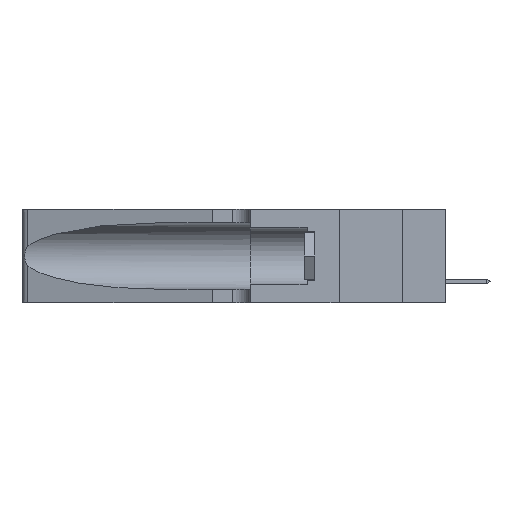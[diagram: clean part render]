
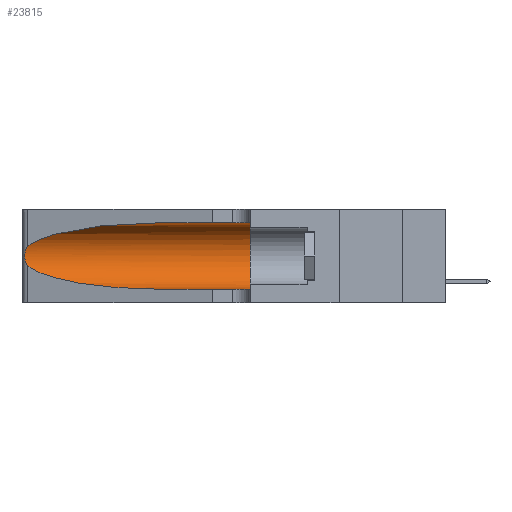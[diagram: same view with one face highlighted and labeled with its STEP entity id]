
A CAD part, left-side view. The second image highlights one B-rep face of the part: STEP entity #23815.
In plain terms, the highlighted cylindrical face has radius 3.308 mm (diameter 6.617 mm), a partial arc.
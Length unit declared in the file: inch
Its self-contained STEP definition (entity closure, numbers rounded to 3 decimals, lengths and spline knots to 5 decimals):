
#308 = CARTESIAN_POINT ( 'NONE',  ( 0.25555, 1.22994, 0.2215 ) ) ;
#346 = EDGE_LOOP ( 'NONE', ( #594, #11282, #1306, #16714, #24257, #5526 ) ) ;
#594 = ORIENTED_EDGE ( 'NONE', *, *, #5024, .T. ) ;
#627 = CARTESIAN_POINT ( 'NONE',  ( 0.26018, 1.23835, 0.19895 ) ) ;
#1306 = ORIENTED_EDGE ( 'NONE', *, *, #1651, .T. ) ;
#1333 = CARTESIAN_POINT ( 'NONE',  ( 0.2373, 1.15595, 0.28018 ) ) ;
#1420 = CARTESIAN_POINT ( 'NONE',  ( 0.25639, 1.23186, 0.15144 ) ) ;
#1492 = CARTESIAN_POINT ( 'NONE',  ( 0.18966, 0.96281, 0.31525 ) ) ;
#1651 = EDGE_CURVE ( 'NONE', #13844, #24138, #10274, .T. ) ;
#1685 = LINE ( 'NONE', #20916, #15355 ) ;
#1821 = CARTESIAN_POINT ( 'NONE',  ( 0.1305, 1.61858, 0.05475 ) ) ;
#2177 = CARTESIAN_POINT ( 'NONE',  ( 0.25789, 1.23486, 0.15765 ) ) ;
#2389 = CARTESIAN_POINT ( 'NONE',  ( 0.1305, 0.35, 0.31525 ) ) ;
#2402 = DIRECTION ( 'NONE',  ( 0., 0., -1. ) ) ;
#3996 = CARTESIAN_POINT ( 'NONE',  ( 0.18966, 0.96281, 0.05475 ) ) ;
#4148 = CARTESIAN_POINT ( 'NONE',  ( 0.25487, 1.22718, 0.14631 ) ) ;
#4607 = VERTEX_POINT ( 'NONE', #18445 ) ;
#4663 = CARTESIAN_POINT ( 'NONE',  ( 0.1305, 0.35, 0.185 ) ) ;
#4810 = EDGE_CURVE ( 'NONE', #20390, #4607, #6855, .T. ) ;
#4836 = DIRECTION ( 'NONE',  ( 0., 0., 1. ) ) ;
#4902 = CARTESIAN_POINT ( 'NONE',  ( 0.25555, 1.22993, 0.14849 ) ) ;
#5024 = EDGE_CURVE ( 'NONE', #6715, #22818, #18009, .T. ) ;
#5433 = DIRECTION ( 'NONE',  ( 0., -1., 0. ) ) ;
#5441 = AXIS2_PLACEMENT_3D ( 'NONE', #4663, #21728, #4836 ) ;
#5526 = ORIENTED_EDGE ( 'NONE', *, *, #13953, .F. ) ;
#5614 = CARTESIAN_POINT ( 'NONE',  ( 0.1305, 0.72297, 0.31525 ) ) ;
#5783 = CARTESIAN_POINT ( 'NONE',  ( 0.25487, 1.22718, 0.22369 ) ) ;
#5871 = CARTESIAN_POINT ( 'NONE',  ( 0.1305, 0.72297, 0.05475 ) ) ;
#6715 = VERTEX_POINT ( 'NONE', #5614 ) ;
#6785 = CARTESIAN_POINT ( 'NONE',  ( 0.1305, 0.72297, 0.05475 ) ) ;
#6855 = CIRCLE ( 'NONE', #5441, 0.13025 ) ;
#8062 = CARTESIAN_POINT ( 'NONE',  ( 0.26075, 1.23896, 0.178 ) ) ;
#9027 = CARTESIAN_POINT ( 'NONE',  ( 0.25487, 1.22718, 0.22369 ) ) ;
#9530 = B_SPLINE_CURVE_WITH_KNOTS ( 'NONE', 3,
 ( #23493, #308, #19420, #17695, #21345, #627, #9800, #8062, #23246, #24098, #2177, #1420, #4902, #12067 ),
 .UNSPECIFIED., .F., .F.,
 ( 4, 2, 2, 2, 2, 2, 4 ),
 ( 0., 0.00027, 0.00053, 0.00107, 0.0016, 0.00187, 0.00214 ),
 .UNSPECIFIED. ) ;
#9800 = CARTESIAN_POINT ( 'NONE',  ( 0.26075, 1.23896, 0.19203 ) ) ;
#10274 =( BOUNDED_CURVE ( )  B_SPLINE_CURVE ( 3, ( #4148, #19191, #3996, #5871 ),
 .UNSPECIFIED., .F., .F. ) 
 B_SPLINE_CURVE_WITH_KNOTS ( ( 4, 4 ),
 ( 3.44316, 4.71239 ),
 .UNSPECIFIED. ) 
 CURVE ( )  GEOMETRIC_REPRESENTATION_ITEM ( )  RATIONAL_B_SPLINE_CURVE ( ( 1., 0.87, 0.87, 1. ) ) 
 REPRESENTATION_ITEM ( '' )  );
#10351 = CYLINDRICAL_SURFACE ( 'NONE', #19291, 0.13025 ) ;
#11282 = ORIENTED_EDGE ( 'NONE', *, *, #15821, .T. ) ;
#11821 = DIRECTION ( 'NONE',  ( 0., -1., 0. ) ) ;
#12067 = CARTESIAN_POINT ( 'NONE',  ( 0.25487, 1.22718, 0.14631 ) ) ;
#13844 = VERTEX_POINT ( 'NONE', #14317 ) ;
#13953 = EDGE_CURVE ( 'NONE', #6715, #20390, #1685, .T. ) ;
#14317 = CARTESIAN_POINT ( 'NONE',  ( 0.25487, 1.22718, 0.14631 ) ) ;
#15355 = VECTOR ( 'NONE', #5433, 39.37008 ) ;
#15545 = CARTESIAN_POINT ( 'NONE',  ( 0.1305, 1.61858, 0.185 ) ) ;
#15821 = EDGE_CURVE ( 'NONE', #22818, #13844, #9530, .T. ) ;
#16479 = CARTESIAN_POINT ( 'NONE',  ( 0.1305, 0.72297, 0.31525 ) ) ;
#16714 = ORIENTED_EDGE ( 'NONE', *, *, #22779, .T. ) ;
#17215 = DIRECTION ( 'NONE',  ( 0., -1., 0. ) ) ;
#17695 = CARTESIAN_POINT ( 'NONE',  ( 0.25787, 1.23484, 0.2124 ) ) ;
#18009 =( BOUNDED_CURVE ( )  B_SPLINE_CURVE ( 3, ( #16479, #1492, #1333, #9027 ),
 .UNSPECIFIED., .F., .F. ) 
 B_SPLINE_CURVE_WITH_KNOTS ( ( 4, 4 ),
 ( 1.5708, 2.84003 ),
 .UNSPECIFIED. ) 
 CURVE ( )  GEOMETRIC_REPRESENTATION_ITEM ( )  RATIONAL_B_SPLINE_CURVE ( ( 1., 0.87, 0.87, 1. ) ) 
 REPRESENTATION_ITEM ( '' )  );
#18445 = CARTESIAN_POINT ( 'NONE',  ( 0.1305, 0.35, 0.05475 ) ) ;
#18869 = LINE ( 'NONE', #1821, #22454 ) ;
#19191 = CARTESIAN_POINT ( 'NONE',  ( 0.2373, 1.15595, 0.08982 ) ) ;
#19291 = AXIS2_PLACEMENT_3D ( 'NONE', #15545, #11821, #2402 ) ;
#19420 = CARTESIAN_POINT ( 'NONE',  ( 0.25639, 1.23184, 0.21858 ) ) ;
#20390 = VERTEX_POINT ( 'NONE', #2389 ) ;
#20916 = CARTESIAN_POINT ( 'NONE',  ( 0.1305, 1.61858, 0.31525 ) ) ;
#21345 = CARTESIAN_POINT ( 'NONE',  ( 0.25854, 1.2359, 0.20912 ) ) ;
#21728 = DIRECTION ( 'NONE',  ( 0., 1., 0. ) ) ;
#22454 = VECTOR ( 'NONE', #17215, 39.37008 ) ;
#22779 = EDGE_CURVE ( 'NONE', #24138, #4607, #18869, .T. ) ;
#22818 = VERTEX_POINT ( 'NONE', #5783 ) ;
#23246 = CARTESIAN_POINT ( 'NONE',  ( 0.26017, 1.23833, 0.17102 ) ) ;
#23493 = CARTESIAN_POINT ( 'NONE',  ( 0.25487, 1.22718, 0.22369 ) ) ;
#23590 = FACE_OUTER_BOUND ( 'NONE', #346, .T. ) ;
#23815 = ADVANCED_FACE ( 'NONE', ( #23590 ), #10351, .F. ) ;
#24098 = CARTESIAN_POINT ( 'NONE',  ( 0.25856, 1.23593, 0.16098 ) ) ;
#24138 = VERTEX_POINT ( 'NONE', #6785 ) ;
#24257 = ORIENTED_EDGE ( 'NONE', *, *, #4810, .F. ) ;
